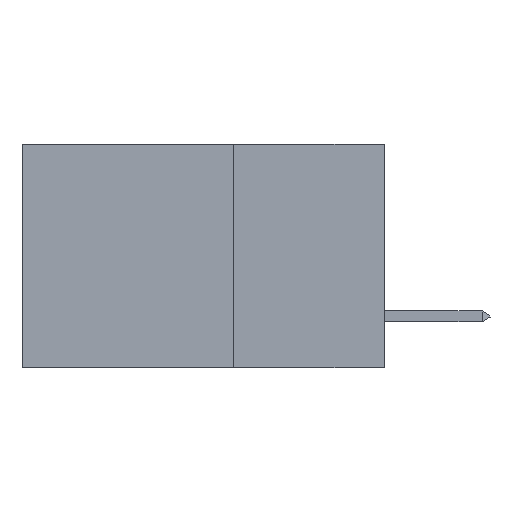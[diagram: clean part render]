
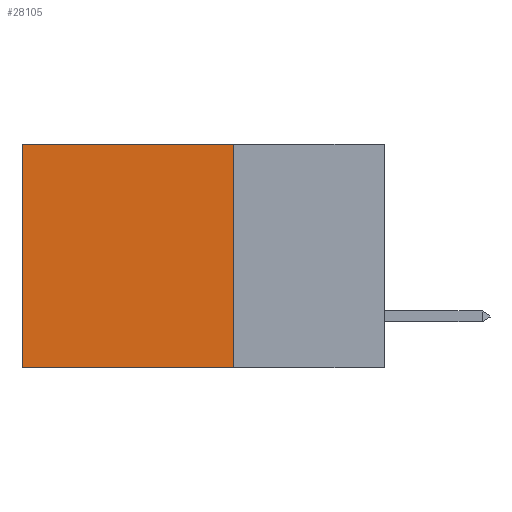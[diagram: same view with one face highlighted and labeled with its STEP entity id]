
A CAD part, left-side view. The second image highlights one B-rep face of the part: STEP entity #28105.
In plain terms, the highlighted planar face has unit normal (-1, 0, 0).
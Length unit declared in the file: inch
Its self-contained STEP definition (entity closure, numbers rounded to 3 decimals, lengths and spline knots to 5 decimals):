
#1325 = DIRECTION ( 'NONE',  ( 0., 0., -1. ) ) ;
#3125 = VERTEX_POINT ( 'NONE', #27834 ) ;
#3782 = VECTOR ( 'NONE', #1325, 39.37008 ) ;
#5663 = VERTEX_POINT ( 'NONE', #37012 ) ;
#5818 = DIRECTION ( 'NONE',  ( 0., 1., 0. ) ) ;
#6992 = CARTESIAN_POINT ( 'NONE',  ( 0.2875, 0.6, 0. ) ) ;
#9896 = LINE ( 'NONE', #21186, #18557 ) ;
#9933 = VERTEX_POINT ( 'NONE', #23893 ) ;
#10626 = PLANE ( 'NONE',  #20806 ) ;
#10976 = VECTOR ( 'NONE', #25043, 39.37008 ) ;
#13301 = EDGE_CURVE ( 'NONE', #5663, #36606, #23745, .T. ) ;
#15046 = ORIENTED_EDGE ( 'NONE', *, *, #21426, .T. ) ;
#15687 = ORIENTED_EDGE ( 'NONE', *, *, #13301, .T. ) ;
#17063 = CARTESIAN_POINT ( 'NONE',  ( 0.2875, 0.6, -0.37 ) ) ;
#17531 = EDGE_LOOP ( 'NONE', ( #15687, #22182, #31758, #15046 ) ) ;
#18511 = EDGE_CURVE ( 'NONE', #3125, #9933, #18851, .T. ) ;
#18557 = VECTOR ( 'NONE', #35899, 39.37008 ) ;
#18851 = LINE ( 'NONE', #36597, #3782 ) ;
#19545 = CARTESIAN_POINT ( 'NONE',  ( 0.2875, 0.25, 0. ) ) ;
#20324 = CARTESIAN_POINT ( 'NONE',  ( 0.2875, 0.25, -0.37 ) ) ;
#20806 = AXIS2_PLACEMENT_3D ( 'NONE', #19545, #25513, #22488 ) ;
#21186 = CARTESIAN_POINT ( 'NONE',  ( 0.2875, 0.25, 0. ) ) ;
#21426 = EDGE_CURVE ( 'NONE', #3125, #5663, #9896, .T. ) ;
#22182 = ORIENTED_EDGE ( 'NONE', *, *, #31793, .F. ) ;
#22488 = DIRECTION ( 'NONE',  ( 0., 0., -1. ) ) ;
#23540 = LINE ( 'NONE', #20324, #37289 ) ;
#23745 = LINE ( 'NONE', #6992, #10976 ) ;
#23893 = CARTESIAN_POINT ( 'NONE',  ( 0.2875, 0.25, -0.37 ) ) ;
#25043 = DIRECTION ( 'NONE',  ( 0., 0., -1. ) ) ;
#25513 = DIRECTION ( 'NONE',  ( 1., 0., 0. ) ) ;
#27834 = CARTESIAN_POINT ( 'NONE',  ( 0.2875, 0.25, 0. ) ) ;
#28105 = ADVANCED_FACE ( 'NONE', ( #31566 ), #10626, .F. ) ;
#31566 = FACE_OUTER_BOUND ( 'NONE', #17531, .T. ) ;
#31758 = ORIENTED_EDGE ( 'NONE', *, *, #18511, .F. ) ;
#31793 = EDGE_CURVE ( 'NONE', #9933, #36606, #23540, .T. ) ;
#35899 = DIRECTION ( 'NONE',  ( 0., 1., 0. ) ) ;
#36597 = CARTESIAN_POINT ( 'NONE',  ( 0.2875, 0.25, 0. ) ) ;
#36606 = VERTEX_POINT ( 'NONE', #17063 ) ;
#37012 = CARTESIAN_POINT ( 'NONE',  ( 0.2875, 0.6, 0. ) ) ;
#37289 = VECTOR ( 'NONE', #5818, 39.37008 ) ;
